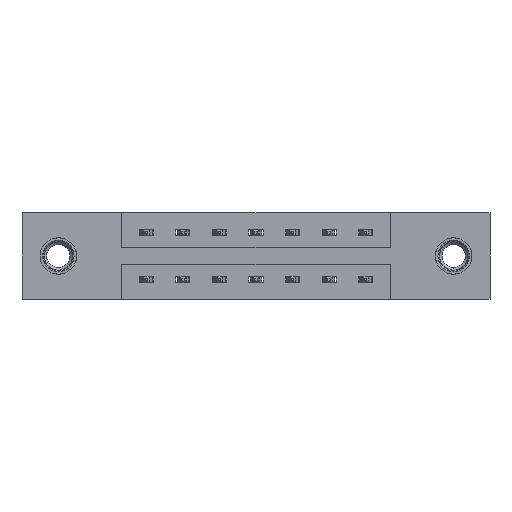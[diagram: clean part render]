
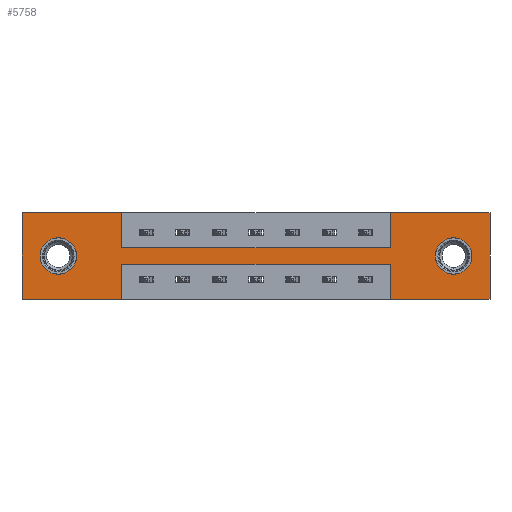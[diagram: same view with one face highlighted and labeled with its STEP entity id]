
A CAD part, front view. The second image highlights one B-rep face of the part: STEP entity #5758.
In plain terms, the highlighted planar face has unit normal (0, -1, 0).
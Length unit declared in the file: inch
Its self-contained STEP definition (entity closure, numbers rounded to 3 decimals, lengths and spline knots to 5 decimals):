
#3 = LINE ( 'NONE', #2285, #8955 ) ;
#72 = FACE_BOUND ( 'NONE', #3401, .T. ) ;
#243 = VERTEX_POINT ( 'NONE', #5661 ) ;
#250 = DIRECTION ( 'NONE',  ( 0., 0., 1. ) ) ;
#300 = VERTEX_POINT ( 'NONE', #2659 ) ;
#325 = VERTEX_POINT ( 'NONE', #3020 ) ;
#500 = CARTESIAN_POINT ( 'NONE',  ( 0.425, 0., 0. ) ) ;
#504 = CARTESIAN_POINT ( 'NONE',  ( 0.425, 0., 0. ) ) ;
#639 = LINE ( 'NONE', #6615, #5012 ) ;
#744 = CARTESIAN_POINT ( 'NONE',  ( 0.155, 0., -0.185 ) ) ;
#1014 = CARTESIAN_POINT ( 'NONE',  ( 0.425, 0., -0.15 ) ) ;
#1070 = CARTESIAN_POINT ( 'NONE',  ( 1.998, 0., 0. ) ) ;
#1081 = CARTESIAN_POINT ( 'NONE',  ( 1.573, 0., -0.37 ) ) ;
#1119 = ORIENTED_EDGE ( 'NONE', *, *, #1150, .F. ) ;
#1150 = EDGE_CURVE ( 'NONE', #4148, #3600, #10469, .T. ) ;
#1239 = CARTESIAN_POINT ( 'NONE',  ( 0.425, 0., -0.15 ) ) ;
#1428 = VERTEX_POINT ( 'NONE', #2965 ) ;
#1487 = VERTEX_POINT ( 'NONE', #1081 ) ;
#1667 = DIRECTION ( 'NONE',  ( 0., 0., 1. ) ) ;
#1804 = VECTOR ( 'NONE', #4587, 39.37008 ) ;
#1837 = ORIENTED_EDGE ( 'NONE', *, *, #2304, .F. ) ;
#1849 = ORIENTED_EDGE ( 'NONE', *, *, #9827, .F. ) ;
#1889 = VERTEX_POINT ( 'NONE', #6657 ) ;
#1916 = LINE ( 'NONE', #5123, #7303 ) ;
#1969 = VERTEX_POINT ( 'NONE', #2144 ) ;
#1997 = CARTESIAN_POINT ( 'NONE',  ( 0., 0., 0. ) ) ;
#2013 = CARTESIAN_POINT ( 'NONE',  ( 1.843, 0., -0.185 ) ) ;
#2041 = EDGE_LOOP ( 'NONE', ( #10367, #3862, #1837, #2124, #9204, #2923, #5228, #7486, #1119, #10257, #10773, #1849 ) ) ;
#2124 = ORIENTED_EDGE ( 'NONE', *, *, #5431, .F. ) ;
#2144 = CARTESIAN_POINT ( 'NONE',  ( 1.573, 0., -0.22 ) ) ;
#2259 = ORIENTED_EDGE ( 'NONE', *, *, #8676, .T. ) ;
#2285 = CARTESIAN_POINT ( 'NONE',  ( 1.573, 0., -0.37 ) ) ;
#2304 = EDGE_CURVE ( 'NONE', #1487, #1969, #3, .T. ) ;
#2604 = VECTOR ( 'NONE', #6661, 39.37008 ) ;
#2659 = CARTESIAN_POINT ( 'NONE',  ( 1.998, 0., 0. ) ) ;
#2756 = DIRECTION ( 'NONE',  ( 0., -1., 0. ) ) ;
#2772 = CARTESIAN_POINT ( 'NONE',  ( 1.573, 0., 0. ) ) ;
#2872 = DIRECTION ( 'NONE',  ( 0., 0., -1. ) ) ;
#2923 = ORIENTED_EDGE ( 'NONE', *, *, #9893, .F. ) ;
#2965 = CARTESIAN_POINT ( 'NONE',  ( 1.998, 0., -0.37 ) ) ;
#2994 = VERTEX_POINT ( 'NONE', #6570 ) ;
#3020 = CARTESIAN_POINT ( 'NONE',  ( 0., 0., -0.37 ) ) ;
#3387 = CARTESIAN_POINT ( 'NONE',  ( 1.843, 0., -0.185 ) ) ;
#3401 = EDGE_LOOP ( 'NONE', ( #7354, #9864 ) ) ;
#3417 = VECTOR ( 'NONE', #4860, 39.37008 ) ;
#3469 = CARTESIAN_POINT ( 'NONE',  ( 1.573, 0., 0. ) ) ;
#3600 = VERTEX_POINT ( 'NONE', #1014 ) ;
#3862 = ORIENTED_EDGE ( 'NONE', *, *, #10078, .F. ) ;
#3958 = CIRCLE ( 'NONE', #7398, 0.078 ) ;
#4009 = DIRECTION ( 'NONE',  ( -1., 0., 0. ) ) ;
#4050 = CIRCLE ( 'NONE', #10423, 0.078 ) ;
#4148 = VERTEX_POINT ( 'NONE', #504 ) ;
#4244 = DIRECTION ( 'NONE',  ( 0., 0., -1. ) ) ;
#4249 = DIRECTION ( 'NONE',  ( 1., 0., 0. ) ) ;
#4257 = ORIENTED_EDGE ( 'NONE', *, *, #7762, .T. ) ;
#4363 = LINE ( 'NONE', #1070, #1804 ) ;
#4440 = CARTESIAN_POINT ( 'NONE',  ( 0., 0., -0.37 ) ) ;
#4496 = VECTOR ( 'NONE', #4009, 39.37008 ) ;
#4527 = CARTESIAN_POINT ( 'NONE',  ( 0.425, 0., -0.22 ) ) ;
#4554 = EDGE_CURVE ( 'NONE', #325, #4606, #8646, .T. ) ;
#4587 = DIRECTION ( 'NONE',  ( 0., 0., -1. ) ) ;
#4606 = VERTEX_POINT ( 'NONE', #5547 ) ;
#4681 = CARTESIAN_POINT ( 'NONE',  ( 0.155, 0., -0.107 ) ) ;
#4758 = FACE_OUTER_BOUND ( 'NONE', #2041, .T. ) ;
#4860 = DIRECTION ( 'NONE',  ( -1., 0., 0. ) ) ;
#4881 = LINE ( 'NONE', #10025, #2604 ) ;
#5012 = VECTOR ( 'NONE', #5762, 39.37008 ) ;
#5024 = CIRCLE ( 'NONE', #7894, 0.078 ) ;
#5035 = VERTEX_POINT ( 'NONE', #6943 ) ;
#5123 = CARTESIAN_POINT ( 'NONE',  ( 0.425, 0., -0.37 ) ) ;
#5126 = VERTEX_POINT ( 'NONE', #2772 ) ;
#5228 = ORIENTED_EDGE ( 'NONE', *, *, #8808, .F. ) ;
#5288 = VERTEX_POINT ( 'NONE', #4681 ) ;
#5431 = EDGE_CURVE ( 'NONE', #1428, #1487, #8774, .T. ) ;
#5525 = DIRECTION ( 'NONE',  ( 0., 1., 0. ) ) ;
#5547 = CARTESIAN_POINT ( 'NONE',  ( 0., 0., 0. ) ) ;
#5661 = CARTESIAN_POINT ( 'NONE',  ( 1.843, 0., -0.107 ) ) ;
#5758 = ADVANCED_FACE ( 'NONE', ( #9296, #72, #4758 ), #7889, .T. ) ;
#5762 = DIRECTION ( 'NONE',  ( -1., 0., 0. ) ) ;
#5952 = EDGE_CURVE ( 'NONE', #3600, #1889, #7436, .T. ) ;
#5982 = VECTOR ( 'NONE', #6304, 39.37008 ) ;
#6107 = VECTOR ( 'NONE', #7176, 39.37008 ) ;
#6115 = DIRECTION ( 'NONE',  ( 0., 0., 1. ) ) ;
#6250 = EDGE_CURVE ( 'NONE', #11092, #9222, #1916, .T. ) ;
#6266 = EDGE_CURVE ( 'NONE', #4606, #4148, #6490, .T. ) ;
#6304 = DIRECTION ( 'NONE',  ( 0., 0., -1. ) ) ;
#6431 = DIRECTION ( 'NONE',  ( 1., 0., 0. ) ) ;
#6490 = LINE ( 'NONE', #10194, #8494 ) ;
#6570 = CARTESIAN_POINT ( 'NONE',  ( 1.843, 0., -0.263 ) ) ;
#6615 = CARTESIAN_POINT ( 'NONE',  ( 0.425, 0., -0.22 ) ) ;
#6657 = CARTESIAN_POINT ( 'NONE',  ( 1.573, 0., -0.15 ) ) ;
#6661 = DIRECTION ( 'NONE',  ( 1., 0., 0. ) ) ;
#6826 = DIRECTION ( 'NONE',  ( 0., 1., 0. ) ) ;
#6870 = AXIS2_PLACEMENT_3D ( 'NONE', #4440, #2756, #8737 ) ;
#6943 = CARTESIAN_POINT ( 'NONE',  ( 0.155, 0., -0.263 ) ) ;
#7175 = VECTOR ( 'NONE', #6115, 39.37008 ) ;
#7176 = DIRECTION ( 'NONE',  ( 0., 0., 1. ) ) ;
#7303 = VECTOR ( 'NONE', #11042, 39.37008 ) ;
#7354 = ORIENTED_EDGE ( 'NONE', *, *, #10848, .T. ) ;
#7398 = AXIS2_PLACEMENT_3D ( 'NONE', #3387, #9363, #4244 ) ;
#7436 = LINE ( 'NONE', #1239, #9152 ) ;
#7486 = ORIENTED_EDGE ( 'NONE', *, *, #5952, .F. ) ;
#7762 = EDGE_CURVE ( 'NONE', #243, #2994, #9323, .T. ) ;
#7889 = PLANE ( 'NONE',  #6870 ) ;
#7894 = AXIS2_PLACEMENT_3D ( 'NONE', #10568, #5525, #250 ) ;
#7962 = LINE ( 'NONE', #8239, #3417 ) ;
#8009 = DIRECTION ( 'NONE',  ( 0., 1., 0. ) ) ;
#8032 = AXIS2_PLACEMENT_3D ( 'NONE', #2013, #8009, #2872 ) ;
#8239 = CARTESIAN_POINT ( 'NONE',  ( 0., 0., -0.37 ) ) ;
#8426 = EDGE_CURVE ( 'NONE', #300, #1428, #4363, .T. ) ;
#8494 = VECTOR ( 'NONE', #4249, 39.37008 ) ;
#8646 = LINE ( 'NONE', #1997, #6107 ) ;
#8676 = EDGE_CURVE ( 'NONE', #2994, #243, #3958, .T. ) ;
#8737 = DIRECTION ( 'NONE',  ( 0., 0., -1. ) ) ;
#8774 = LINE ( 'NONE', #9967, #4496 ) ;
#8808 = EDGE_CURVE ( 'NONE', #1889, #5126, #8886, .T. ) ;
#8886 = LINE ( 'NONE', #3469, #7175 ) ;
#8955 = VECTOR ( 'NONE', #9189, 39.37008 ) ;
#9152 = VECTOR ( 'NONE', #6431, 39.37008 ) ;
#9189 = DIRECTION ( 'NONE',  ( 0., 0., 1. ) ) ;
#9204 = ORIENTED_EDGE ( 'NONE', *, *, #8426, .F. ) ;
#9222 = VERTEX_POINT ( 'NONE', #10006 ) ;
#9296 = FACE_BOUND ( 'NONE', #9786, .T. ) ;
#9323 = CIRCLE ( 'NONE', #8032, 0.078 ) ;
#9363 = DIRECTION ( 'NONE',  ( 0., 1., 0. ) ) ;
#9667 = EDGE_CURVE ( 'NONE', #5035, #5288, #5024, .T. ) ;
#9786 = EDGE_LOOP ( 'NONE', ( #4257, #2259 ) ) ;
#9827 = EDGE_CURVE ( 'NONE', #9222, #325, #7962, .T. ) ;
#9864 = ORIENTED_EDGE ( 'NONE', *, *, #9667, .T. ) ;
#9893 = EDGE_CURVE ( 'NONE', #5126, #300, #4881, .T. ) ;
#9967 = CARTESIAN_POINT ( 'NONE',  ( 0., 0., -0.37 ) ) ;
#10006 = CARTESIAN_POINT ( 'NONE',  ( 0.425, 0., -0.37 ) ) ;
#10025 = CARTESIAN_POINT ( 'NONE',  ( 0., 0., 0. ) ) ;
#10078 = EDGE_CURVE ( 'NONE', #1969, #11092, #639, .T. ) ;
#10194 = CARTESIAN_POINT ( 'NONE',  ( 0., 0., 0. ) ) ;
#10257 = ORIENTED_EDGE ( 'NONE', *, *, #6266, .F. ) ;
#10367 = ORIENTED_EDGE ( 'NONE', *, *, #6250, .F. ) ;
#10423 = AXIS2_PLACEMENT_3D ( 'NONE', #744, #6826, #1667 ) ;
#10469 = LINE ( 'NONE', #500, #5982 ) ;
#10568 = CARTESIAN_POINT ( 'NONE',  ( 0.155, 0., -0.185 ) ) ;
#10773 = ORIENTED_EDGE ( 'NONE', *, *, #4554, .F. ) ;
#10848 = EDGE_CURVE ( 'NONE', #5288, #5035, #4050, .T. ) ;
#11042 = DIRECTION ( 'NONE',  ( 0., 0., -1. ) ) ;
#11092 = VERTEX_POINT ( 'NONE', #4527 ) ;
